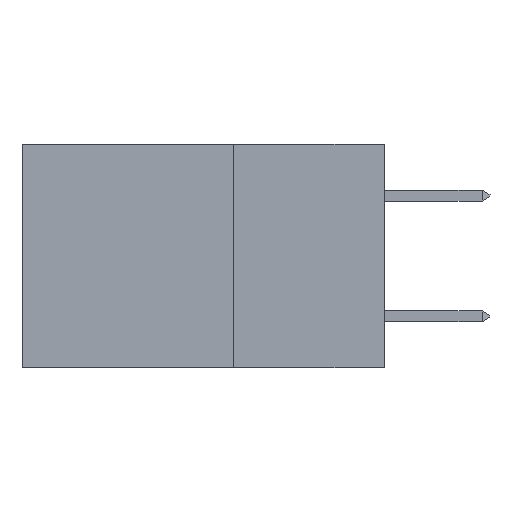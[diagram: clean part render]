
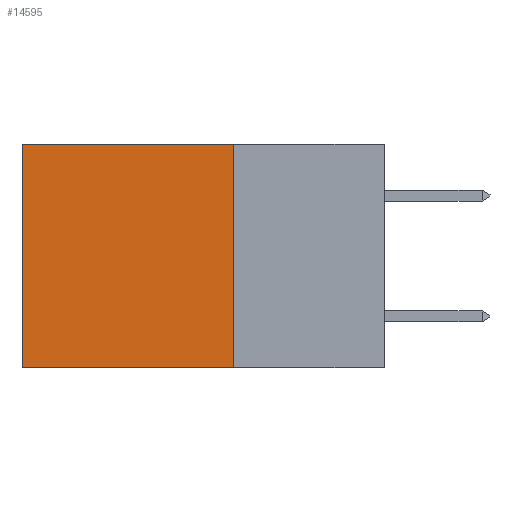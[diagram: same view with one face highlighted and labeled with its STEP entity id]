
A CAD part, left-side view. The second image highlights one B-rep face of the part: STEP entity #14595.
In plain terms, the highlighted planar face has unit normal (-1, 0, 0).
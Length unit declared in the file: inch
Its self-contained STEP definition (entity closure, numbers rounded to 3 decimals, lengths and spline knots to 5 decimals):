
#571 = CARTESIAN_POINT ( 'NONE',  ( 0.2875, 0.25, 0. ) ) ;
#1948 = VECTOR ( 'NONE', #10210, 39.37008 ) ;
#3016 = DIRECTION ( 'NONE',  ( 1., 0., 0. ) ) ;
#4142 = LINE ( 'NONE', #4681, #8448 ) ;
#4256 = CARTESIAN_POINT ( 'NONE',  ( 0.2875, 0.25, -0.37 ) ) ;
#4681 = CARTESIAN_POINT ( 'NONE',  ( 0.2875, 0.6, 0. ) ) ;
#5191 = LINE ( 'NONE', #6556, #1948 ) ;
#5376 = DIRECTION ( 'NONE',  ( 0., 0., -1. ) ) ;
#5755 = VERTEX_POINT ( 'NONE', #6554 ) ;
#5788 = CARTESIAN_POINT ( 'NONE',  ( 0.2875, 0.6, 0. ) ) ;
#6554 = CARTESIAN_POINT ( 'NONE',  ( 0.2875, 0.25, 0. ) ) ;
#6556 = CARTESIAN_POINT ( 'NONE',  ( 0.2875, 0.25, 0. ) ) ;
#6576 = PLANE ( 'NONE',  #13063 ) ;
#6735 = ORIENTED_EDGE ( 'NONE', *, *, #9002, .T. ) ;
#6764 = DIRECTION ( 'NONE',  ( 0., 1., 0. ) ) ;
#6766 = VECTOR ( 'NONE', #15463, 39.37008 ) ;
#7584 = FACE_OUTER_BOUND ( 'NONE', #14539, .T. ) ;
#7971 = EDGE_CURVE ( 'NONE', #11094, #11865, #8734, .T. ) ;
#8380 = EDGE_CURVE ( 'NONE', #5755, #11094, #11802, .T. ) ;
#8390 = CARTESIAN_POINT ( 'NONE',  ( 0.2875, 0.6, -0.37 ) ) ;
#8448 = VECTOR ( 'NONE', #13391, 39.37008 ) ;
#8734 = LINE ( 'NONE', #4256, #15767 ) ;
#9002 = EDGE_CURVE ( 'NONE', #5755, #12385, #5191, .T. ) ;
#10027 = CARTESIAN_POINT ( 'NONE',  ( 0.2875, 0.25, -0.37 ) ) ;
#10210 = DIRECTION ( 'NONE',  ( 0., 1., 0. ) ) ;
#10420 = ORIENTED_EDGE ( 'NONE', *, *, #8380, .F. ) ;
#11094 = VERTEX_POINT ( 'NONE', #10027 ) ;
#11240 = EDGE_CURVE ( 'NONE', #12385, #11865, #4142, .T. ) ;
#11802 = LINE ( 'NONE', #571, #6766 ) ;
#11865 = VERTEX_POINT ( 'NONE', #8390 ) ;
#12385 = VERTEX_POINT ( 'NONE', #5788 ) ;
#13063 = AXIS2_PLACEMENT_3D ( 'NONE', #15413, #3016, #5376 ) ;
#13326 = ORIENTED_EDGE ( 'NONE', *, *, #11240, .T. ) ;
#13391 = DIRECTION ( 'NONE',  ( 0., 0., -1. ) ) ;
#14539 = EDGE_LOOP ( 'NONE', ( #13326, #14948, #10420, #6735 ) ) ;
#14595 = ADVANCED_FACE ( 'NONE', ( #7584 ), #6576, .F. ) ;
#14948 = ORIENTED_EDGE ( 'NONE', *, *, #7971, .F. ) ;
#15413 = CARTESIAN_POINT ( 'NONE',  ( 0.2875, 0.25, 0. ) ) ;
#15463 = DIRECTION ( 'NONE',  ( 0., 0., -1. ) ) ;
#15767 = VECTOR ( 'NONE', #6764, 39.37008 ) ;
